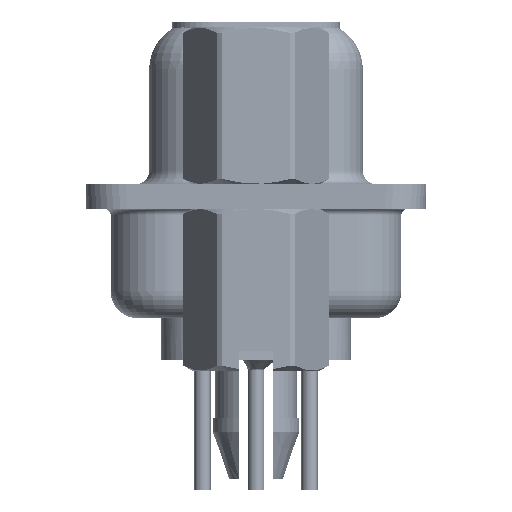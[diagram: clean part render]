
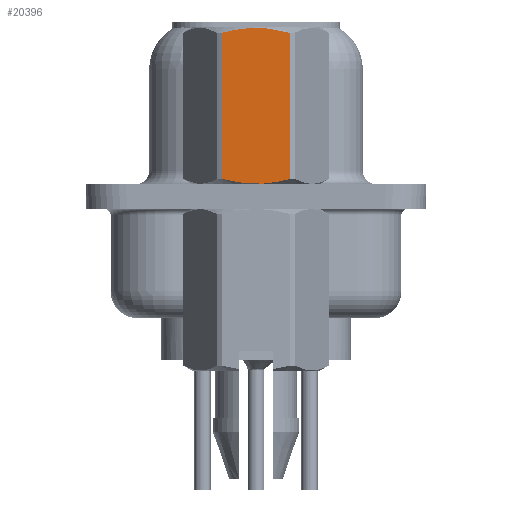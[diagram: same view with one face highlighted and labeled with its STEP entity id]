
A CAD part, left-side view. The second image highlights one B-rep face of the part: STEP entity #20396.
In plain terms, the highlighted planar face has unit normal (-1, 0, 0).
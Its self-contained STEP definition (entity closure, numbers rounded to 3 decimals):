
#1413 = ORIENTED_EDGE ( 'NONE', *, *, #28977, .T. ) ;
#1540 = VECTOR ( 'NONE', #13958, 1000. ) ;
#1548 = B_SPLINE_CURVE_WITH_KNOTS ( 'NONE', 3,
 ( #26147, #11249, #38328, #29488, #2620, #20271, #8129, #32618, #38511, #20075 ),
 .UNSPECIFIED., .F., .F.,
 ( 4, 2, 2, 2, 4 ),
 ( 0.001, 0.002, 0.002, 0.003, 0.004 ),
 .UNSPECIFIED. ) ;
#2482 = CARTESIAN_POINT ( 'NONE',  ( -2.381, -1.066, 0.596 ) ) ;
#2620 = CARTESIAN_POINT ( 'NONE',  ( -2.381, -0.215, 6.232 ) ) ;
#3780 = CARTESIAN_POINT ( 'NONE',  ( -2.381, 1.375, -3.75 ) ) ;
#4310 = CARTESIAN_POINT ( 'NONE',  ( -2.381, -1.273, 6.048 ) ) ;
#4997 = CARTESIAN_POINT ( 'NONE',  ( -2.381, 1.273, 0.652 ) ) ;
#5252 = B_SPLINE_CURVE_WITH_KNOTS ( 'NONE', 3,
 ( #12079, #17369, #26964, #14432, #24026, #9148, #29347, #33040, #2482, #35598 ),
 .UNSPECIFIED., .F., .F.,
 ( 4, 2, 2, 2, 4 ),
 ( 0.003, 0.003, 0.004, 0.004, 0.005 ),
 .UNSPECIFIED. ) ;
#6923 = DIRECTION ( 'NONE',  ( -1., 0., 0. ) ) ;
#7423 = AXIS2_PLACEMENT_3D ( 'NONE', #3780, #6923, #18867 ) ;
#8129 = CARTESIAN_POINT ( 'NONE',  ( -2.381, 0.428, 6.215 ) ) ;
#9148 = CARTESIAN_POINT ( 'NONE',  ( -2.381, -0.215, 0.468 ) ) ;
#10921 = EDGE_CURVE ( 'NONE', #36793, #24673, #5252, .T. ) ;
#11249 = CARTESIAN_POINT ( 'NONE',  ( -2.381, -1.066, 6.104 ) ) ;
#11588 = LINE ( 'NONE', #16894, #1540 ) ;
#12079 = CARTESIAN_POINT ( 'NONE',  ( -2.381, 1.273, 0.652 ) ) ;
#12086 = EDGE_LOOP ( 'NONE', ( #12214, #23281, #27697, #1413 ) ) ;
#12209 = PLANE ( 'NONE',  #7423 ) ;
#12214 = ORIENTED_EDGE ( 'NONE', *, *, #10921, .T. ) ;
#13958 = DIRECTION ( 'NONE',  ( 0., 0., -1. ) ) ;
#14432 = CARTESIAN_POINT ( 'NONE',  ( -2.381, 0.428, 0.485 ) ) ;
#14933 = FACE_OUTER_BOUND ( 'NONE', #12086, .T. ) ;
#16894 = CARTESIAN_POINT ( 'NONE',  ( -2.381, 1.273, 3.792 ) ) ;
#17369 = CARTESIAN_POINT ( 'NONE',  ( -2.381, 1.065, 0.596 ) ) ;
#18867 = DIRECTION ( 'NONE',  ( 0., -1., 0. ) ) ;
#20075 = CARTESIAN_POINT ( 'NONE',  ( -2.381, 1.273, 6.048 ) ) ;
#20271 = CARTESIAN_POINT ( 'NONE',  ( -2.381, 0.215, 6.232 ) ) ;
#20396 = ADVANCED_FACE ( 'NONE', ( #14933 ), #12209, .T. ) ;
#22004 = DIRECTION ( 'NONE',  ( 0., 0., 1. ) ) ;
#22386 = LINE ( 'NONE', #34344, #31996 ) ;
#23240 = EDGE_CURVE ( 'NONE', #24673, #29183, #22386, .T. ) ;
#23281 = ORIENTED_EDGE ( 'NONE', *, *, #23240, .T. ) ;
#24026 = CARTESIAN_POINT ( 'NONE',  ( -2.381, 0.215, 0.468 ) ) ;
#24673 = VERTEX_POINT ( 'NONE', #27935 ) ;
#25071 = CARTESIAN_POINT ( 'NONE',  ( -2.381, 1.273, 6.048 ) ) ;
#26147 = CARTESIAN_POINT ( 'NONE',  ( -2.381, -1.273, 6.048 ) ) ;
#26964 = CARTESIAN_POINT ( 'NONE',  ( -2.381, 0.853, 0.549 ) ) ;
#27697 = ORIENTED_EDGE ( 'NONE', *, *, #28545, .T. ) ;
#27935 = CARTESIAN_POINT ( 'NONE',  ( -2.381, -1.273, 0.652 ) ) ;
#28545 = EDGE_CURVE ( 'NONE', #29183, #33621, #1548, .T. ) ;
#28977 = EDGE_CURVE ( 'NONE', #33621, #36793, #11588, .T. ) ;
#29183 = VERTEX_POINT ( 'NONE', #4310 ) ;
#29347 = CARTESIAN_POINT ( 'NONE',  ( -2.381, -0.432, 0.485 ) ) ;
#29488 = CARTESIAN_POINT ( 'NONE',  ( -2.381, -0.432, 6.215 ) ) ;
#31996 = VECTOR ( 'NONE', #22004, 1000. ) ;
#32618 = CARTESIAN_POINT ( 'NONE',  ( -2.381, 0.853, 6.151 ) ) ;
#33040 = CARTESIAN_POINT ( 'NONE',  ( -2.381, -0.858, 0.55 ) ) ;
#33621 = VERTEX_POINT ( 'NONE', #25071 ) ;
#34344 = CARTESIAN_POINT ( 'NONE',  ( -2.381, -1.273, 3.792 ) ) ;
#35598 = CARTESIAN_POINT ( 'NONE',  ( -2.381, -1.273, 0.652 ) ) ;
#36793 = VERTEX_POINT ( 'NONE', #4997 ) ;
#38328 = CARTESIAN_POINT ( 'NONE',  ( -2.381, -0.858, 6.15 ) ) ;
#38511 = CARTESIAN_POINT ( 'NONE',  ( -2.381, 1.065, 6.104 ) ) ;
